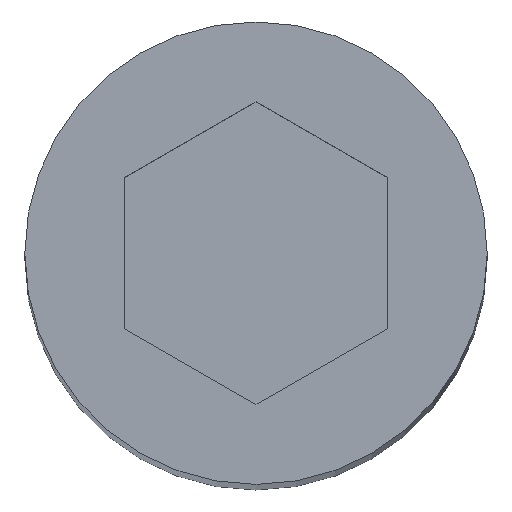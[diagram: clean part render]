
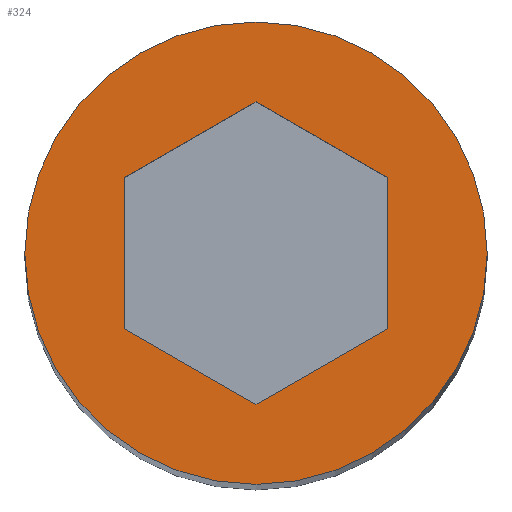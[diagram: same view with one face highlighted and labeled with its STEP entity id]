
A CAD part, top view. The second image highlights one B-rep face of the part: STEP entity #324.
In plain terms, the highlighted planar face has unit normal (0, 0, 1).
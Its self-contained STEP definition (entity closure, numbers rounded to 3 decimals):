
#3 = CARTESIAN_POINT ( 'NONE',  ( 2.125, 1.227, 52.25 ) ) ;
#7 = DIRECTION ( 'NONE',  ( 1., 0., 0. ) ) ;
#12 = CARTESIAN_POINT ( 'NONE',  ( -2.125, -1.227, 52.25 ) ) ;
#16 = CARTESIAN_POINT ( 'NONE',  ( 2.125, 1.227, 52.25 ) ) ;
#22 = DIRECTION ( 'NONE',  ( 1., 0., 0. ) ) ;
#24 = EDGE_CURVE ( 'NONE', #214, #229, #123, .T. ) ;
#26 = DIRECTION ( 'NONE',  ( 0., 1., 0. ) ) ;
#27 = CARTESIAN_POINT ( 'NONE',  ( 2.125, -1.227, 52.25 ) ) ;
#32 = CARTESIAN_POINT ( 'NONE',  ( 0., -2.454, 52.25 ) ) ;
#33 = DIRECTION ( 'NONE',  ( 0.866, 0.5, 0. ) ) ;
#35 = CARTESIAN_POINT ( 'NONE',  ( -2.125, 1.227, 52.25 ) ) ;
#48 = CARTESIAN_POINT ( 'NONE',  ( 0., -2.454, 52.25 ) ) ;
#59 = EDGE_CURVE ( 'NONE', #295, #279, #115, .T. ) ;
#68 = PLANE ( 'NONE',  #335 ) ;
#69 = EDGE_CURVE ( 'NONE', #273, #342, #230, .T. ) ;
#80 = CARTESIAN_POINT ( 'NONE',  ( 0., 2.454, 52.25 ) ) ;
#81 = CARTESIAN_POINT ( 'NONE',  ( 2.125, -1.227, 52.25 ) ) ;
#83 = CARTESIAN_POINT ( 'NONE',  ( 0., 0., 52.25 ) ) ;
#88 = AXIS2_PLACEMENT_3D ( 'NONE', #126, #113, #112 ) ;
#89 = EDGE_CURVE ( 'NONE', #346, #215, #144, .T. ) ;
#92 = DIRECTION ( 'NONE',  ( -0.866, -0.5, 0. ) ) ;
#93 = VECTOR ( 'NONE', #33, 1000. ) ;
#96 = CARTESIAN_POINT ( 'NONE',  ( 0., 2.454, 52.25 ) ) ;
#97 = VECTOR ( 'NONE', #26, 1000. ) ;
#105 = DIRECTION ( 'NONE',  ( -0.866, 0.5, 0. ) ) ;
#107 = DIRECTION ( 'NONE',  ( 0., 0., 1. ) ) ;
#112 = DIRECTION ( 'NONE',  ( 1., 0., 0. ) ) ;
#113 = DIRECTION ( 'NONE',  ( 0., 0., 1. ) ) ;
#115 = CIRCLE ( 'NONE', #88, 3.75 ) ;
#122 = DIRECTION ( 'NONE',  ( 0., 0., 1. ) ) ;
#123 = LINE ( 'NONE', #27, #97 ) ;
#126 = CARTESIAN_POINT ( 'NONE',  ( 0., 0., 52.25 ) ) ;
#144 = LINE ( 'NONE', #12, #264 ) ;
#145 = EDGE_CURVE ( 'NONE', #342, #346, #181, .T. ) ;
#158 = DIRECTION ( 'NONE',  ( 0., -1., 0. ) ) ;
#159 = CARTESIAN_POINT ( 'NONE',  ( -2.125, 1.227, 52.25 ) ) ;
#162 = CARTESIAN_POINT ( 'NONE',  ( -3.75, 0., 52.25 ) ) ;
#165 = FACE_BOUND ( 'NONE', #235, .T. ) ;
#166 = CIRCLE ( 'NONE', #339, 3.75 ) ;
#167 = FACE_OUTER_BOUND ( 'NONE', #253, .T. ) ;
#169 = LINE ( 'NONE', #48, #93 ) ;
#179 = LINE ( 'NONE', #16, #180 ) ;
#180 = VECTOR ( 'NONE', #105, 1000. ) ;
#181 = LINE ( 'NONE', #159, #183 ) ;
#183 = VECTOR ( 'NONE', #158, 1000. ) ;
#205 = CARTESIAN_POINT ( 'NONE',  ( 3.75, 0., 52.25 ) ) ;
#210 = CARTESIAN_POINT ( 'NONE',  ( -2.125, -1.227, 52.25 ) ) ;
#214 = VERTEX_POINT ( 'NONE', #81 ) ;
#215 = VERTEX_POINT ( 'NONE', #32 ) ;
#225 = EDGE_CURVE ( 'NONE', #229, #273, #179, .T. ) ;
#229 = VERTEX_POINT ( 'NONE', #3 ) ;
#230 = LINE ( 'NONE', #96, #261 ) ;
#235 = EDGE_LOOP ( 'NONE', ( #327, #296, #275, #318, #303, #280 ) ) ;
#237 = ORIENTED_EDGE ( 'NONE', *, *, #313, .T. ) ;
#253 = EDGE_LOOP ( 'NONE', ( #237, #284 ) ) ;
#261 = VECTOR ( 'NONE', #92, 1000. ) ;
#264 = VECTOR ( 'NONE', #321, 1000. ) ;
#273 = VERTEX_POINT ( 'NONE', #80 ) ;
#275 = ORIENTED_EDGE ( 'NONE', *, *, #276, .F. ) ;
#276 = EDGE_CURVE ( 'NONE', #215, #214, #169, .T. ) ;
#279 = VERTEX_POINT ( 'NONE', #162 ) ;
#280 = ORIENTED_EDGE ( 'NONE', *, *, #69, .F. ) ;
#284 = ORIENTED_EDGE ( 'NONE', *, *, #59, .T. ) ;
#295 = VERTEX_POINT ( 'NONE', #205 ) ;
#296 = ORIENTED_EDGE ( 'NONE', *, *, #24, .F. ) ;
#303 = ORIENTED_EDGE ( 'NONE', *, *, #145, .F. ) ;
#313 = EDGE_CURVE ( 'NONE', #279, #295, #166, .T. ) ;
#318 = ORIENTED_EDGE ( 'NONE', *, *, #89, .F. ) ;
#319 = CARTESIAN_POINT ( 'NONE',  ( 0., 0., 52.25 ) ) ;
#321 = DIRECTION ( 'NONE',  ( 0.866, -0.5, 0. ) ) ;
#324 = ADVANCED_FACE ( 'NONE', ( #165, #167 ), #68, .T. ) ;
#327 = ORIENTED_EDGE ( 'NONE', *, *, #225, .F. ) ;
#335 = AXIS2_PLACEMENT_3D ( 'NONE', #83, #122, #22 ) ;
#339 = AXIS2_PLACEMENT_3D ( 'NONE', #319, #107, #7 ) ;
#342 = VERTEX_POINT ( 'NONE', #35 ) ;
#346 = VERTEX_POINT ( 'NONE', #210 ) ;
